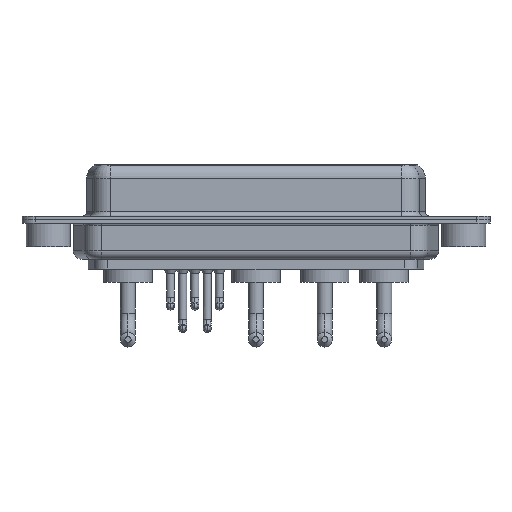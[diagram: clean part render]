
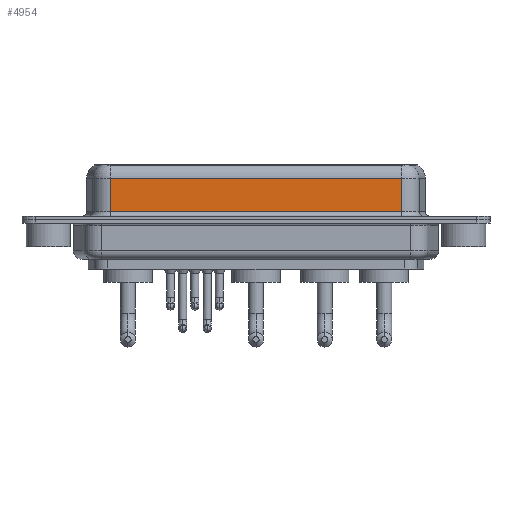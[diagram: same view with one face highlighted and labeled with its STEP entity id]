
A CAD part, front view. The second image highlights one B-rep face of the part: STEP entity #4954.
In plain terms, the highlighted planar face has unit normal (0, -1, 0).
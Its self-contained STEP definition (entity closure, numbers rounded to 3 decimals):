
#166 = LINE ( 'NONE', #5143, #2885 ) ;
#803 = PLANE ( 'NONE',  #16485 ) ;
#1237 = CARTESIAN_POINT ( 'NONE',  ( 7.013, -3.95, 0.9 ) ) ;
#1797 = VERTEX_POINT ( 'NONE', #5799 ) ;
#2161 = VERTEX_POINT ( 'NONE', #1237 ) ;
#2671 = EDGE_CURVE ( 'NONE', #8449, #2161, #16258, .T. ) ;
#2885 = VECTOR ( 'NONE', #10787, 1000. ) ;
#4120 = ORIENTED_EDGE ( 'NONE', *, *, #7522, .T. ) ;
#4448 = VECTOR ( 'NONE', #7332, 1000. ) ;
#4469 = EDGE_LOOP ( 'NONE', ( #5426, #4120, #10903, #10755 ) ) ;
#4954 = ADVANCED_FACE ( 'NONE', ( #10027 ), #803, .F. ) ;
#5143 = CARTESIAN_POINT ( 'NONE',  ( 40.037, -3.95, 4.65 ) ) ;
#5426 = ORIENTED_EDGE ( 'NONE', *, *, #6817, .F. ) ;
#5706 = CARTESIAN_POINT ( 'NONE',  ( 40.037, -3.95, 4.65 ) ) ;
#5799 = CARTESIAN_POINT ( 'NONE',  ( 40.037, -3.95, 0.9 ) ) ;
#5805 = VERTEX_POINT ( 'NONE', #5706 ) ;
#6817 = EDGE_CURVE ( 'NONE', #5805, #1797, #12961, .T. ) ;
#7332 = DIRECTION ( 'NONE',  ( 0., 0., -1. ) ) ;
#7378 = VECTOR ( 'NONE', #7908, 1000. ) ;
#7522 = EDGE_CURVE ( 'NONE', #5805, #8449, #166, .T. ) ;
#7816 = LINE ( 'NONE', #17226, #7378 ) ;
#7908 = DIRECTION ( 'NONE',  ( 1., 0., 0. ) ) ;
#8449 = VERTEX_POINT ( 'NONE', #16403 ) ;
#9546 = CARTESIAN_POINT ( 'NONE',  ( 7.013, -3.95, 6.4 ) ) ;
#10027 = FACE_OUTER_BOUND ( 'NONE', #4469, .T. ) ;
#10755 = ORIENTED_EDGE ( 'NONE', *, *, #13598, .T. ) ;
#10787 = DIRECTION ( 'NONE',  ( -1., 0., 0. ) ) ;
#10903 = ORIENTED_EDGE ( 'NONE', *, *, #2671, .T. ) ;
#11494 = DIRECTION ( 'NONE',  ( 0., 1., 0. ) ) ;
#12541 = CARTESIAN_POINT ( 'NONE',  ( 40.037, -3.95, 6.4 ) ) ;
#12961 = LINE ( 'NONE', #14199, #4448 ) ;
#13000 = VECTOR ( 'NONE', #13469, 1000. ) ;
#13469 = DIRECTION ( 'NONE',  ( 0., 0., -1. ) ) ;
#13598 = EDGE_CURVE ( 'NONE', #2161, #1797, #7816, .T. ) ;
#14199 = CARTESIAN_POINT ( 'NONE',  ( 40.037, -3.95, 6.4 ) ) ;
#16258 = LINE ( 'NONE', #9546, #13000 ) ;
#16403 = CARTESIAN_POINT ( 'NONE',  ( 7.013, -3.95, 4.65 ) ) ;
#16485 = AXIS2_PLACEMENT_3D ( 'NONE', #12541, #11494, #16652 ) ;
#16652 = DIRECTION ( 'NONE',  ( 0., 0., 1. ) ) ;
#17226 = CARTESIAN_POINT ( 'NONE',  ( 40.037, -3.95, 0.9 ) ) ;
